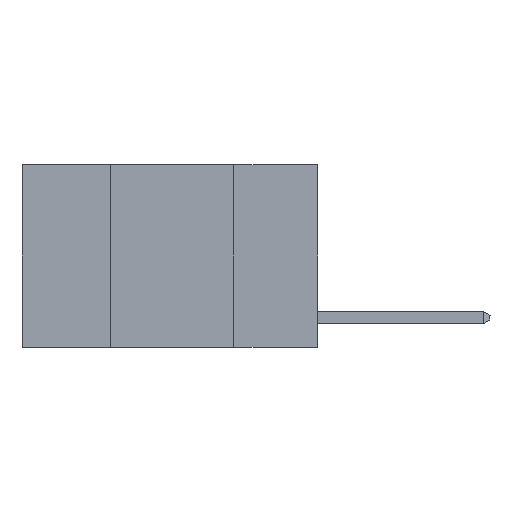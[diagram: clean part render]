
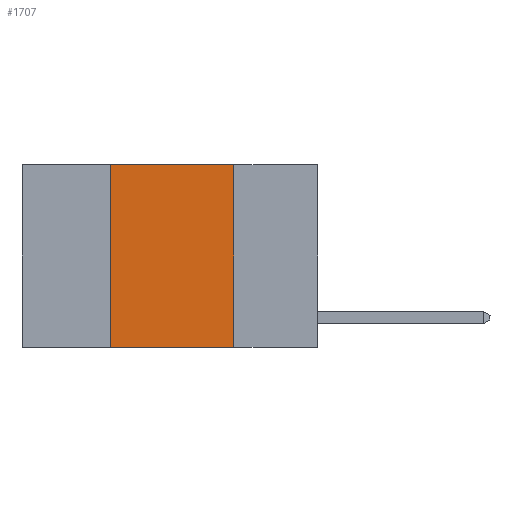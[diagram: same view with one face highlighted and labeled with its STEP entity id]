
A CAD part, left-side view. The second image highlights one B-rep face of the part: STEP entity #1707.
In plain terms, the highlighted planar face has unit normal (-1, 0, 0).
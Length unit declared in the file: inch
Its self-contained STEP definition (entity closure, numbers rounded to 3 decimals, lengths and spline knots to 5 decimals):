
#554 = EDGE_CURVE ( 'NONE', #7161, #5288, #3362, .T. ) ;
#694 = ORIENTED_EDGE ( 'NONE', *, *, #5675, .F. ) ;
#1185 = DIRECTION ( 'NONE',  ( 1., 0., 0. ) ) ;
#1244 = DIRECTION ( 'NONE',  ( 0., 0., -1. ) ) ;
#1707 = ADVANCED_FACE ( 'NONE', ( #12394 ), #10663, .F. ) ;
#1913 = DIRECTION ( 'NONE',  ( 0., -1., 0. ) ) ;
#2287 = VECTOR ( 'NONE', #5963, 39.37008 ) ;
#2780 = VERTEX_POINT ( 'NONE', #13737 ) ;
#3062 = DIRECTION ( 'NONE',  ( 0., 0., -1. ) ) ;
#3362 = LINE ( 'NONE', #11478, #10735 ) ;
#4035 = EDGE_LOOP ( 'NONE', ( #7084, #13489, #694, #6217 ) ) ;
#4901 = LINE ( 'NONE', #7689, #13348 ) ;
#5288 = VERTEX_POINT ( 'NONE', #8129 ) ;
#5675 = EDGE_CURVE ( 'NONE', #2780, #11277, #9002, .T. ) ;
#5963 = DIRECTION ( 'NONE',  ( 0., 0., 1. ) ) ;
#6125 = EDGE_CURVE ( 'NONE', #11277, #7161, #10516, .T. ) ;
#6153 = EDGE_CURVE ( 'NONE', #2780, #5288, #4901, .T. ) ;
#6217 = ORIENTED_EDGE ( 'NONE', *, *, #6153, .T. ) ;
#6293 = CARTESIAN_POINT ( 'NONE',  ( 0., 0.6, 0. ) ) ;
#6352 = DIRECTION ( 'NONE',  ( 0., -1., 0. ) ) ;
#7029 = CARTESIAN_POINT ( 'NONE',  ( 0., 0.42, 0. ) ) ;
#7084 = ORIENTED_EDGE ( 'NONE', *, *, #554, .F. ) ;
#7161 = VERTEX_POINT ( 'NONE', #14609 ) ;
#7689 = CARTESIAN_POINT ( 'NONE',  ( 0., 0.6, -0.37 ) ) ;
#8129 = CARTESIAN_POINT ( 'NONE',  ( 0., 0.17, -0.37 ) ) ;
#8929 = CARTESIAN_POINT ( 'NONE',  ( 0., 0.42, 0. ) ) ;
#8987 = VECTOR ( 'NONE', #1913, 39.37008 ) ;
#9002 = LINE ( 'NONE', #8929, #2287 ) ;
#10516 = LINE ( 'NONE', #6293, #8987 ) ;
#10663 = PLANE ( 'NONE',  #14308 ) ;
#10735 = VECTOR ( 'NONE', #3062, 39.37008 ) ;
#11277 = VERTEX_POINT ( 'NONE', #7029 ) ;
#11478 = CARTESIAN_POINT ( 'NONE',  ( 0., 0.17, 0. ) ) ;
#12394 = FACE_OUTER_BOUND ( 'NONE', #4035, .T. ) ;
#13348 = VECTOR ( 'NONE', #6352, 39.37008 ) ;
#13489 = ORIENTED_EDGE ( 'NONE', *, *, #6125, .F. ) ;
#13737 = CARTESIAN_POINT ( 'NONE',  ( 0., 0.42, -0.37 ) ) ;
#14308 = AXIS2_PLACEMENT_3D ( 'NONE', #15071, #1185, #1244 ) ;
#14609 = CARTESIAN_POINT ( 'NONE',  ( 0., 0.17, 0. ) ) ;
#15071 = CARTESIAN_POINT ( 'NONE',  ( 0., 0.6, 0. ) ) ;
